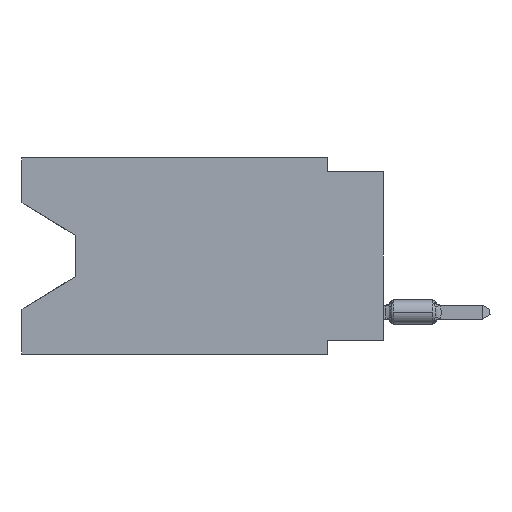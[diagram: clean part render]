
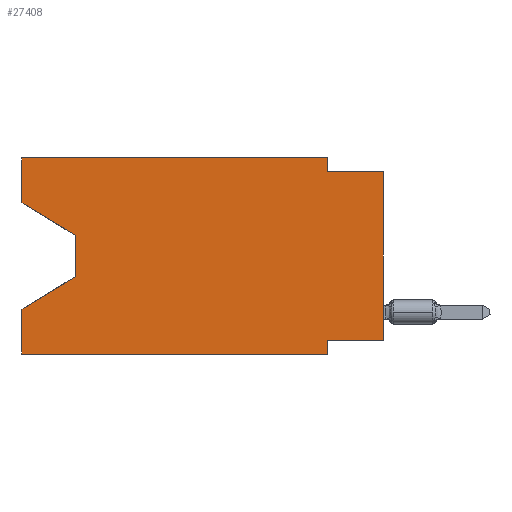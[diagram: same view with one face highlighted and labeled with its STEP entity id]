
A CAD part, left-side view. The second image highlights one B-rep face of the part: STEP entity #27408.
In plain terms, the highlighted planar face has unit normal (-1, 0, 0).
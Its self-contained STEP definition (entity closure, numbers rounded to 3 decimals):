
#233 = LINE ( 'NONE', #76213, #27302 ) ;
#1433 = CARTESIAN_POINT ( 'NONE',  ( 0., 0., 0. ) ) ;
#2582 = CARTESIAN_POINT ( 'NONE',  ( 0., 16.383, -6.852 ) ) ;
#3657 = LINE ( 'NONE', #75019, #79300 ) ;
#5264 = VECTOR ( 'NONE', #81609, 1000. ) ;
#5546 = EDGE_LOOP ( 'NONE', ( #33906, #46124, #18125, #41166, #72419, #60151, #69447, #5828, #12873, #37765, #61222, #31029 ) ) ;
#5828 = ORIENTED_EDGE ( 'NONE', *, *, #39318, .T. ) ;
#6653 = VERTEX_POINT ( 'NONE', #2582 ) ;
#6966 = VERTEX_POINT ( 'NONE', #82695 ) ;
#8151 = DIRECTION ( 'NONE',  ( 0., 0., 1. ) ) ;
#9150 = DIRECTION ( 'NONE',  ( 0., 0., 1. ) ) ;
#10038 = DIRECTION ( 'NONE',  ( 0., -1., 0. ) ) ;
#11635 = VERTEX_POINT ( 'NONE', #67714 ) ;
#12142 = CARTESIAN_POINT ( 'NONE',  ( 0., 2.54, -0.635 ) ) ;
#12278 = CARTESIAN_POINT ( 'NONE',  ( 0., 16.383, 0. ) ) ;
#12873 = ORIENTED_EDGE ( 'NONE', *, *, #14582, .F. ) ;
#13032 = LINE ( 'NONE', #26054, #74375 ) ;
#13622 = EDGE_CURVE ( 'NONE', #16876, #57916, #62491, .T. ) ;
#14582 = EDGE_CURVE ( 'NONE', #47750, #35505, #81180, .T. ) ;
#16876 = VERTEX_POINT ( 'NONE', #73377 ) ;
#17251 = LINE ( 'NONE', #22720, #21076 ) ;
#18125 = ORIENTED_EDGE ( 'NONE', *, *, #78469, .T. ) ;
#19532 = DIRECTION ( 'NONE',  ( 0., 0.855, -0.519 ) ) ;
#21076 = VECTOR ( 'NONE', #47495, 1000. ) ;
#21816 = CARTESIAN_POINT ( 'NONE',  ( 0., 2.54, -8.89 ) ) ;
#22720 = CARTESIAN_POINT ( 'NONE',  ( 0., 16.383, -2.038 ) ) ;
#23396 = VERTEX_POINT ( 'NONE', #78763 ) ;
#23687 = CARTESIAN_POINT ( 'NONE',  ( 0., 0., -0.635 ) ) ;
#24357 = EDGE_CURVE ( 'NONE', #61859, #26473, #17251, .T. ) ;
#24594 = DIRECTION ( 'NONE',  ( 0., -1., 0. ) ) ;
#25286 = PLANE ( 'NONE',  #63002 ) ;
#26054 = CARTESIAN_POINT ( 'NONE',  ( 0., 2.54, 0. ) ) ;
#26473 = VERTEX_POINT ( 'NONE', #78115 ) ;
#27302 = VECTOR ( 'NONE', #19532, 1000. ) ;
#27408 = ADVANCED_FACE ( 'NONE', ( #64300 ), #25286, .F. ) ;
#27445 = LINE ( 'NONE', #1433, #39310 ) ;
#28224 = VECTOR ( 'NONE', #37779, 1000. ) ;
#29219 = VECTOR ( 'NONE', #10038, 1000. ) ;
#31029 = ORIENTED_EDGE ( 'NONE', *, *, #49097, .F. ) ;
#32773 = VECTOR ( 'NONE', #37694, 1000. ) ;
#33049 = EDGE_CURVE ( 'NONE', #57916, #47750, #13032, .T. ) ;
#33062 = LINE ( 'NONE', #65817, #73563 ) ;
#33906 = ORIENTED_EDGE ( 'NONE', *, *, #24357, .T. ) ;
#34791 = EDGE_CURVE ( 'NONE', #11635, #60479, #53735, .T. ) ;
#34819 = DIRECTION ( 'NONE',  ( 0., 0., -1. ) ) ;
#35212 = CARTESIAN_POINT ( 'NONE',  ( 0., 16.383, 0. ) ) ;
#35505 = VERTEX_POINT ( 'NONE', #58067 ) ;
#37580 = EDGE_CURVE ( 'NONE', #23396, #60479, #82090, .T. ) ;
#37694 = DIRECTION ( 'NONE',  ( 0., 0., -1. ) ) ;
#37765 = ORIENTED_EDGE ( 'NONE', *, *, #33049, .F. ) ;
#37779 = DIRECTION ( 'NONE',  ( 0., 1., 0. ) ) ;
#39310 = VECTOR ( 'NONE', #8151, 1000. ) ;
#39318 = EDGE_CURVE ( 'NONE', #71186, #35505, #27445, .T. ) ;
#39860 = DIRECTION ( 'NONE',  ( 0., 0., -1. ) ) ;
#41128 = EDGE_CURVE ( 'NONE', #26473, #6966, #70826, .T. ) ;
#41166 = ORIENTED_EDGE ( 'NONE', *, *, #82633, .F. ) ;
#44070 = CARTESIAN_POINT ( 'NONE',  ( 0., 0., -8.255 ) ) ;
#45160 = CARTESIAN_POINT ( 'NONE',  ( 0., 16.383, -2.038 ) ) ;
#46124 = ORIENTED_EDGE ( 'NONE', *, *, #41128, .T. ) ;
#47495 = DIRECTION ( 'NONE',  ( 0., -0.855, -0.519 ) ) ;
#47750 = VERTEX_POINT ( 'NONE', #12142 ) ;
#49097 = EDGE_CURVE ( 'NONE', #61859, #16876, #3657, .T. ) ;
#49364 = CARTESIAN_POINT ( 'NONE',  ( 0., 16.383, -8.89 ) ) ;
#51487 = CARTESIAN_POINT ( 'NONE',  ( 0., 0., -8.255 ) ) ;
#53735 = LINE ( 'NONE', #21816, #67902 ) ;
#57460 = DIRECTION ( 'NONE',  ( 0., 0., 1. ) ) ;
#57605 = DIRECTION ( 'NONE',  ( 0., 0., -1. ) ) ;
#57916 = VERTEX_POINT ( 'NONE', #61849 ) ;
#58067 = CARTESIAN_POINT ( 'NONE',  ( 0., 0., -0.635 ) ) ;
#60151 = ORIENTED_EDGE ( 'NONE', *, *, #34791, .F. ) ;
#60479 = VERTEX_POINT ( 'NONE', #72090 ) ;
#61222 = ORIENTED_EDGE ( 'NONE', *, *, #13622, .F. ) ;
#61849 = CARTESIAN_POINT ( 'NONE',  ( 0., 2.54, 0. ) ) ;
#61859 = VERTEX_POINT ( 'NONE', #45160 ) ;
#62491 = LINE ( 'NONE', #35212, #29219 ) ;
#63002 = AXIS2_PLACEMENT_3D ( 'NONE', #12278, #76071, #57605 ) ;
#64300 = FACE_OUTER_BOUND ( 'NONE', #5546, .T. ) ;
#65817 = CARTESIAN_POINT ( 'NONE',  ( 0., 16.383, 0. ) ) ;
#67714 = CARTESIAN_POINT ( 'NONE',  ( 0., 2.54, -8.255 ) ) ;
#67902 = VECTOR ( 'NONE', #34819, 1000. ) ;
#68016 = VECTOR ( 'NONE', #24594, 1000. ) ;
#68843 = LINE ( 'NONE', #44070, #28224 ) ;
#68983 = EDGE_CURVE ( 'NONE', #71186, #11635, #68843, .T. ) ;
#69447 = ORIENTED_EDGE ( 'NONE', *, *, #68983, .F. ) ;
#70826 = LINE ( 'NONE', #77134, #32773 ) ;
#71186 = VERTEX_POINT ( 'NONE', #51487 ) ;
#72090 = CARTESIAN_POINT ( 'NONE',  ( 0., 2.54, -8.89 ) ) ;
#72419 = ORIENTED_EDGE ( 'NONE', *, *, #37580, .T. ) ;
#73377 = CARTESIAN_POINT ( 'NONE',  ( 0., 16.383, 0. ) ) ;
#73563 = VECTOR ( 'NONE', #57460, 1000. ) ;
#74375 = VECTOR ( 'NONE', #39860, 1000. ) ;
#75019 = CARTESIAN_POINT ( 'NONE',  ( 0., 16.383, 0. ) ) ;
#76071 = DIRECTION ( 'NONE',  ( 1., 0., 0. ) ) ;
#76213 = CARTESIAN_POINT ( 'NONE',  ( 0., 13.97, -5.385 ) ) ;
#77134 = CARTESIAN_POINT ( 'NONE',  ( 0., 13.97, -3.505 ) ) ;
#78115 = CARTESIAN_POINT ( 'NONE',  ( 0., 13.97, -3.505 ) ) ;
#78469 = EDGE_CURVE ( 'NONE', #6966, #6653, #233, .T. ) ;
#78763 = CARTESIAN_POINT ( 'NONE',  ( 0., 16.383, -8.89 ) ) ;
#79300 = VECTOR ( 'NONE', #9150, 1000. ) ;
#81180 = LINE ( 'NONE', #23687, #5264 ) ;
#81609 = DIRECTION ( 'NONE',  ( 0., -1., 0. ) ) ;
#82090 = LINE ( 'NONE', #49364, #68016 ) ;
#82633 = EDGE_CURVE ( 'NONE', #23396, #6653, #33062, .T. ) ;
#82695 = CARTESIAN_POINT ( 'NONE',  ( 0., 13.97, -5.385 ) ) ;
